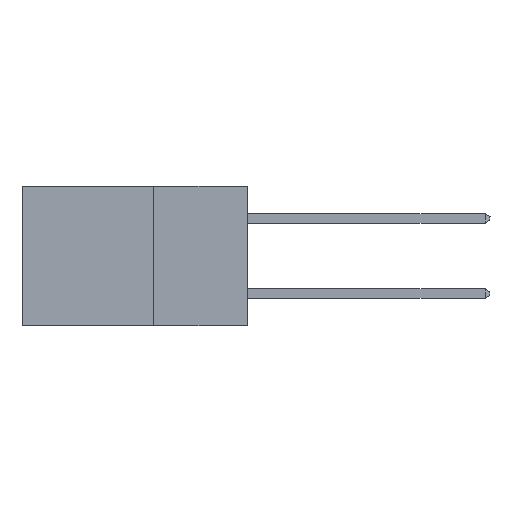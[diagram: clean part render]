
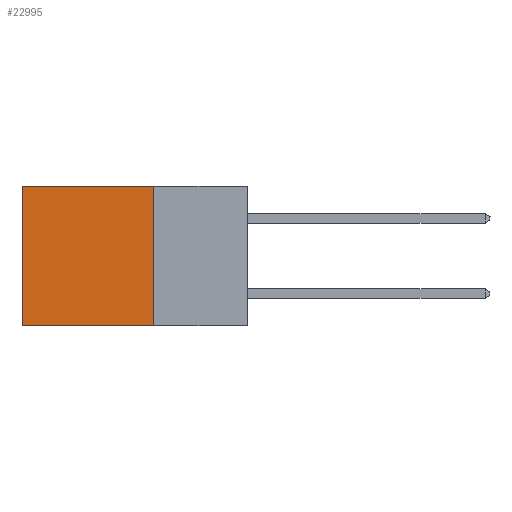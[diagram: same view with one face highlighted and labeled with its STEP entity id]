
A CAD part, left-side view. The second image highlights one B-rep face of the part: STEP entity #22995.
In plain terms, the highlighted planar face has unit normal (-1, 0, 0).
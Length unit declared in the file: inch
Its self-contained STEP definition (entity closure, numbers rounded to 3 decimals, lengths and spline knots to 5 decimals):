
#2185 = CARTESIAN_POINT ( 'NONE',  ( 0.2615, 0.25, -0.37 ) ) ;
#2463 = CARTESIAN_POINT ( 'NONE',  ( 0.2615, 0.6, -0.37 ) ) ;
#2735 = CARTESIAN_POINT ( 'NONE',  ( 0.2615, 0.6, 0. ) ) ;
#2758 = VECTOR ( 'NONE', #7044, 39.37008 ) ;
#3230 = ORIENTED_EDGE ( 'NONE', *, *, #16048, .T. ) ;
#3615 = EDGE_CURVE ( 'NONE', #14659, #13525, #17991, .T. ) ;
#4061 = DIRECTION ( 'NONE',  ( 1., 0., 0. ) ) ;
#5207 = DIRECTION ( 'NONE',  ( 0., 0., -1. ) ) ;
#5330 = CARTESIAN_POINT ( 'NONE',  ( 0.2615, 0.25, -0.37 ) ) ;
#5989 = AXIS2_PLACEMENT_3D ( 'NONE', #11502, #4061, #23143 ) ;
#6429 = EDGE_CURVE ( 'NONE', #12696, #18053, #13103, .T. ) ;
#6434 = VECTOR ( 'NONE', #5207, 39.37008 ) ;
#7044 = DIRECTION ( 'NONE',  ( 0., 0., -1. ) ) ;
#8803 = EDGE_CURVE ( 'NONE', #13525, #18053, #22096, .T. ) ;
#10273 = ORIENTED_EDGE ( 'NONE', *, *, #3615, .F. ) ;
#11178 = VECTOR ( 'NONE', #16626, 39.37008 ) ;
#11502 = CARTESIAN_POINT ( 'NONE',  ( 0.2615, 0.25, -0.37 ) ) ;
#12696 = VERTEX_POINT ( 'NONE', #2735 ) ;
#13103 = LINE ( 'NONE', #16711, #2758 ) ;
#13525 = VERTEX_POINT ( 'NONE', #2185 ) ;
#14618 = CARTESIAN_POINT ( 'NONE',  ( 0.2615, 0.25, 0. ) ) ;
#14659 = VERTEX_POINT ( 'NONE', #14618 ) ;
#14750 = CARTESIAN_POINT ( 'NONE',  ( 0.2615, 0.25, 0. ) ) ;
#15577 = PLANE ( 'NONE',  #5989 ) ;
#16048 = EDGE_CURVE ( 'NONE', #14659, #12696, #24170, .T. ) ;
#16626 = DIRECTION ( 'NONE',  ( 0., 1., 0. ) ) ;
#16682 = ORIENTED_EDGE ( 'NONE', *, *, #8803, .F. ) ;
#16711 = CARTESIAN_POINT ( 'NONE',  ( 0.2615, 0.6, -0.37 ) ) ;
#17991 = LINE ( 'NONE', #24074, #6434 ) ;
#18053 = VERTEX_POINT ( 'NONE', #2463 ) ;
#19897 = ORIENTED_EDGE ( 'NONE', *, *, #6429, .T. ) ;
#21284 = FACE_OUTER_BOUND ( 'NONE', #22656, .T. ) ;
#22075 = VECTOR ( 'NONE', #22310, 39.37008 ) ;
#22096 = LINE ( 'NONE', #5330, #11178 ) ;
#22310 = DIRECTION ( 'NONE',  ( 0., 1., 0. ) ) ;
#22656 = EDGE_LOOP ( 'NONE', ( #19897, #16682, #10273, #3230 ) ) ;
#22995 = ADVANCED_FACE ( 'NONE', ( #21284 ), #15577, .F. ) ;
#23143 = DIRECTION ( 'NONE',  ( 0., 0., -1. ) ) ;
#24074 = CARTESIAN_POINT ( 'NONE',  ( 0.2615, 0.25, -0.37 ) ) ;
#24170 = LINE ( 'NONE', #14750, #22075 ) ;
